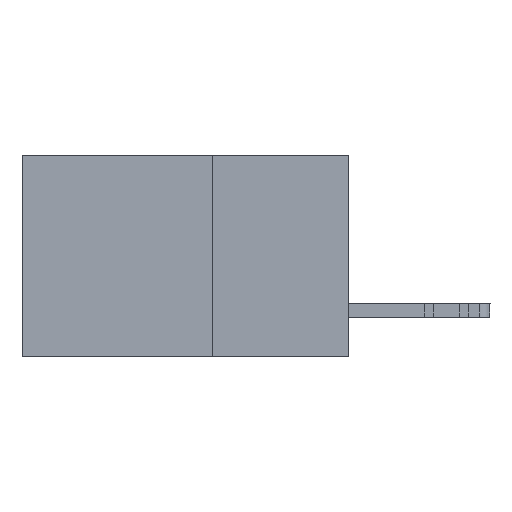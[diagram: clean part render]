
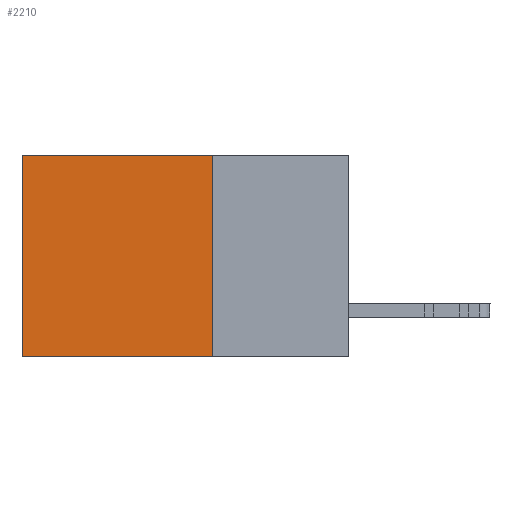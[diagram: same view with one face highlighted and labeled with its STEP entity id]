
A CAD part, left-side view. The second image highlights one B-rep face of the part: STEP entity #2210.
In plain terms, the highlighted planar face has unit normal (-1, 0, 0).
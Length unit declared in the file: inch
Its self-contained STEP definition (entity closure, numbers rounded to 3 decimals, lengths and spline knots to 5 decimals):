
#1179 = DIRECTION ( 'NONE',  ( 1., 0., 0. ) ) ;
#1644 = LINE ( 'NONE', #1991, #11233 ) ;
#1705 = CARTESIAN_POINT ( 'NONE',  ( 0.2615, 0.25, -0.37 ) ) ;
#1991 = CARTESIAN_POINT ( 'NONE',  ( 0.2615, 0.25, -0.37 ) ) ;
#2210 = ADVANCED_FACE ( 'NONE', ( #2954 ), #10329, .F. ) ;
#2848 = ORIENTED_EDGE ( 'NONE', *, *, #19453, .F. ) ;
#2954 = FACE_OUTER_BOUND ( 'NONE', #10122, .T. ) ;
#3183 = DIRECTION ( 'NONE',  ( 0., 0., -1. ) ) ;
#3299 = DIRECTION ( 'NONE',  ( 0., 1., 0. ) ) ;
#4179 = VERTEX_POINT ( 'NONE', #10666 ) ;
#5082 = CARTESIAN_POINT ( 'NONE',  ( 0.2615, 0.25, 0. ) ) ;
#5356 = DIRECTION ( 'NONE',  ( 0., 1., 0. ) ) ;
#5375 = LINE ( 'NONE', #1705, #19884 ) ;
#6747 = VECTOR ( 'NONE', #3183, 39.37008 ) ;
#8688 = EDGE_CURVE ( 'NONE', #22999, #13251, #5375, .T. ) ;
#10122 = EDGE_LOOP ( 'NONE', ( #15441, #2848, #19534, #20565 ) ) ;
#10329 = PLANE ( 'NONE',  #22255 ) ;
#10450 = CARTESIAN_POINT ( 'NONE',  ( 0.2615, 0.25, -0.37 ) ) ;
#10666 = CARTESIAN_POINT ( 'NONE',  ( 0.2615, 0.6, -0.37 ) ) ;
#10984 = VERTEX_POINT ( 'NONE', #17374 ) ;
#11233 = VECTOR ( 'NONE', #3299, 39.37008 ) ;
#13251 = VERTEX_POINT ( 'NONE', #10450 ) ;
#14279 = DIRECTION ( 'NONE',  ( 0., 0., -1. ) ) ;
#14596 = CARTESIAN_POINT ( 'NONE',  ( 0.2615, 0.25, 0. ) ) ;
#14722 = LINE ( 'NONE', #14596, #22613 ) ;
#15441 = ORIENTED_EDGE ( 'NONE', *, *, #22907, .T. ) ;
#15661 = DIRECTION ( 'NONE',  ( 0., 0., -1. ) ) ;
#17374 = CARTESIAN_POINT ( 'NONE',  ( 0.2615, 0.6, 0. ) ) ;
#17444 = CARTESIAN_POINT ( 'NONE',  ( 0.2615, 0.25, -0.37 ) ) ;
#19343 = LINE ( 'NONE', #19457, #6747 ) ;
#19453 = EDGE_CURVE ( 'NONE', #13251, #4179, #1644, .T. ) ;
#19457 = CARTESIAN_POINT ( 'NONE',  ( 0.2615, 0.6, -0.37 ) ) ;
#19534 = ORIENTED_EDGE ( 'NONE', *, *, #8688, .F. ) ;
#19884 = VECTOR ( 'NONE', #14279, 39.37008 ) ;
#20242 = EDGE_CURVE ( 'NONE', #22999, #10984, #14722, .T. ) ;
#20565 = ORIENTED_EDGE ( 'NONE', *, *, #20242, .T. ) ;
#22255 = AXIS2_PLACEMENT_3D ( 'NONE', #17444, #1179, #15661 ) ;
#22613 = VECTOR ( 'NONE', #5356, 39.37008 ) ;
#22907 = EDGE_CURVE ( 'NONE', #10984, #4179, #19343, .T. ) ;
#22999 = VERTEX_POINT ( 'NONE', #5082 ) ;
